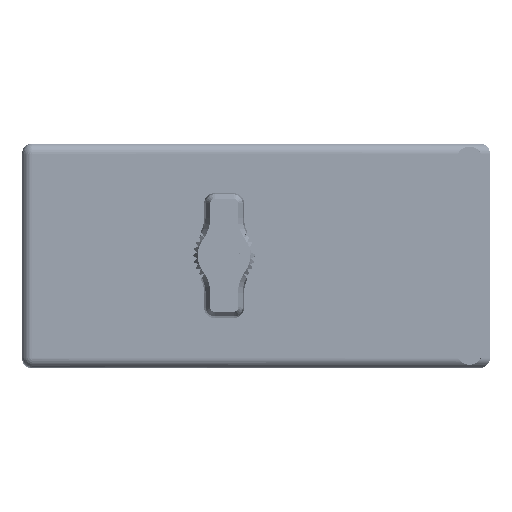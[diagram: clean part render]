
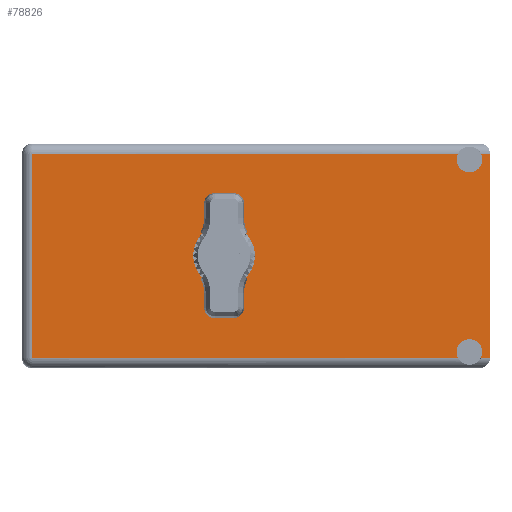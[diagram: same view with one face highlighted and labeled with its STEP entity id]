
A CAD part, top view. The second image highlights one B-rep face of the part: STEP entity #78826.
In plain terms, the highlighted face is planar.
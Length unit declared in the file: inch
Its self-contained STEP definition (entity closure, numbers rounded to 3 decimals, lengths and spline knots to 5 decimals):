
#187 = AXIS2_PLACEMENT_3D ( 'NONE', #57638, #48033, #14824 ) ;
#410 = CARTESIAN_POINT ( 'NONE',  ( 3.05, 2.03, -0.109 ) ) ;
#473 = VECTOR ( 'NONE', #90902, 39.37008 ) ;
#3218 = CARTESIAN_POINT ( 'NONE',  ( 2.97167, 2.03, -0.07 ) ) ;
#3903 = CARTESIAN_POINT ( 'NONE',  ( 3.19, 2.03, -0.07 ) ) ;
#4873 = CARTESIAN_POINT ( 'NONE',  ( 3.05, 2.03, -0.109 ) ) ;
#5989 = AXIS2_PLACEMENT_3D ( 'NONE', #103078, #86810, #69148 ) ;
#7048 = LINE ( 'NONE', #72676, #58517 ) ;
#9829 = DIRECTION ( 'NONE',  ( 1., 0., 0. ) ) ;
#10785 = DIRECTION ( 'NONE',  ( 0., 0., 1. ) ) ;
#13335 = DIRECTION ( 'NONE',  ( 0., 0., 1. ) ) ;
#13415 = VERTEX_POINT ( 'NONE', #73515 ) ;
#14133 = CIRCLE ( 'NONE', #187, 0.17 ) ;
#14623 = CIRCLE ( 'NONE', #77875, 0.0875 ) ;
#14824 = DIRECTION ( 'NONE',  ( 0., 0., 1. ) ) ;
#17156 = ORIENTED_EDGE ( 'NONE', *, *, #49502, .T. ) ;
#18059 = LINE ( 'NONE', #3903, #64268 ) ;
#18221 = VERTEX_POINT ( 'NONE', #25398 ) ;
#20281 = EDGE_CURVE ( 'NONE', #93238, #92271, #7048, .T. ) ;
#22033 = DIRECTION ( 'NONE',  ( 0., 0., 1. ) ) ;
#24570 = DIRECTION ( 'NONE',  ( 0., 1., 0. ) ) ;
#25398 = CARTESIAN_POINT ( 'NONE',  ( 1.3775, 2.03, -0.935 ) ) ;
#25740 = CARTESIAN_POINT ( 'NONE',  ( 2.97167, 2.03, -1.46 ) ) ;
#26006 = EDGE_CURVE ( 'NONE', #99739, #13415, #52169, .T. ) ;
#29541 = VERTEX_POINT ( 'NONE', #3218 ) ;
#31482 = CARTESIAN_POINT ( 'NONE',  ( 1.3775, 2.03, -0.595 ) ) ;
#32822 = CARTESIAN_POINT ( 'NONE',  ( 3.19, 2.03, -0.07 ) ) ;
#33106 = DIRECTION ( 'NONE',  ( 0., 1., 0. ) ) ;
#33468 = EDGE_CURVE ( 'NONE', #92677, #103857, #14623, .T. ) ;
#34198 = CARTESIAN_POINT ( 'NONE',  ( 3.19, 2.03, -0.07 ) ) ;
#34290 = ORIENTED_EDGE ( 'NONE', *, *, #36029, .F. ) ;
#36029 = EDGE_CURVE ( 'NONE', #13415, #29541, #36387, .T. ) ;
#36302 = AXIS2_PLACEMENT_3D ( 'NONE', #75220, #33106, #92182 ) ;
#36387 = CIRCLE ( 'NONE', #49057, 0.0875 ) ;
#36665 = EDGE_CURVE ( 'NONE', #18221, #41378, #106216, .T. ) ;
#36980 = DIRECTION ( 'NONE',  ( -1., 0., 0. ) ) ;
#37032 = CARTESIAN_POINT ( 'NONE',  ( 3.05, 2.03, -1.3335 ) ) ;
#37826 = DIRECTION ( 'NONE',  ( 1., 0., 0. ) ) ;
#40071 = CARTESIAN_POINT ( 'NONE',  ( 0.07, 2.03, -0.07 ) ) ;
#41191 = EDGE_LOOP ( 'NONE', ( #17156, #34290, #84764, #99276, #94895, #71056, #51616, #69160, #60393, #68053 ) ) ;
#41378 = VERTEX_POINT ( 'NONE', #31482 ) ;
#41881 = VECTOR ( 'NONE', #10785, 39.37008 ) ;
#44046 = AXIS2_PLACEMENT_3D ( 'NONE', #98160, #57509, #74173 ) ;
#45121 = CARTESIAN_POINT ( 'NONE',  ( 0., 2.03, -1.46 ) ) ;
#48033 = DIRECTION ( 'NONE',  ( 0., 1., 0. ) ) ;
#48607 = EDGE_CURVE ( 'NONE', #90953, #93238, #75284, .T. ) ;
#49057 = AXIS2_PLACEMENT_3D ( 'NONE', #410, #93023, #51255 ) ;
#49502 = EDGE_CURVE ( 'NONE', #92271, #29541, #81591, .T. ) ;
#49671 = CARTESIAN_POINT ( 'NONE',  ( 3.05, 2.03, -1.421 ) ) ;
#50411 = EDGE_CURVE ( 'NONE', #41378, #18221, #14133, .T. ) ;
#50850 = EDGE_CURVE ( 'NONE', #95085, #96416, #64353, .T. ) ;
#51255 = DIRECTION ( 'NONE',  ( 0., 0., 1. ) ) ;
#51616 = ORIENTED_EDGE ( 'NONE', *, *, #33468, .F. ) ;
#51783 = FACE_OUTER_BOUND ( 'NONE', #41191, .T. ) ;
#52169 = CIRCLE ( 'NONE', #99230, 0.0875 ) ;
#56058 = CARTESIAN_POINT ( 'NONE',  ( 0.07, 2.03, -1.46 ) ) ;
#57509 = DIRECTION ( 'NONE',  ( 0., 1., 0. ) ) ;
#57638 = CARTESIAN_POINT ( 'NONE',  ( 1.3775, 2.03, -0.765 ) ) ;
#58517 = VECTOR ( 'NONE', #22033, 39.37008 ) ;
#58681 = EDGE_LOOP ( 'NONE', ( #77665, #72167 ) ) ;
#60339 = CARTESIAN_POINT ( 'NONE',  ( 3.12833, 2.03, -0.07 ) ) ;
#60393 = ORIENTED_EDGE ( 'NONE', *, *, #48607, .T. ) ;
#63176 = VECTOR ( 'NONE', #9829, 39.37008 ) ;
#63917 = DIRECTION ( 'NONE',  ( 0., 1., 0. ) ) ;
#64268 = VECTOR ( 'NONE', #37826, 39.37008 ) ;
#64353 = LINE ( 'NONE', #103118, #41881 ) ;
#68053 = ORIENTED_EDGE ( 'NONE', *, *, #20281, .T. ) ;
#69148 = DIRECTION ( 'NONE',  ( 0., 0., 1. ) ) ;
#69160 = ORIENTED_EDGE ( 'NONE', *, *, #107006, .F. ) ;
#71056 = ORIENTED_EDGE ( 'NONE', *, *, #78273, .T. ) ;
#71354 = EDGE_CURVE ( 'NONE', #99739, #96416, #18059, .T. ) ;
#72167 = ORIENTED_EDGE ( 'NONE', *, *, #36665, .F. ) ;
#72676 = CARTESIAN_POINT ( 'NONE',  ( 0.07, 2.03, -1.53 ) ) ;
#73515 = CARTESIAN_POINT ( 'NONE',  ( 3.05, 2.03, -0.1965 ) ) ;
#73583 = CARTESIAN_POINT ( 'NONE',  ( 3.12833, 2.03, -1.46 ) ) ;
#74173 = DIRECTION ( 'NONE',  ( 0., 0., 1. ) ) ;
#75220 = CARTESIAN_POINT ( 'NONE',  ( 1.3775, 2.03, -0.765 ) ) ;
#75284 = LINE ( 'NONE', #45121, #99112 ) ;
#75439 = CARTESIAN_POINT ( 'NONE',  ( 3.19, 2.03, -1.46 ) ) ;
#77665 = ORIENTED_EDGE ( 'NONE', *, *, #50411, .F. ) ;
#77875 = AXIS2_PLACEMENT_3D ( 'NONE', #49671, #24570, #83646 ) ;
#78273 = EDGE_CURVE ( 'NONE', #95085, #103857, #102142, .T. ) ;
#78826 = ADVANCED_FACE ( 'NONE', ( #105946, #51783 ), #106634, .T. ) ;
#81591 = LINE ( 'NONE', #34198, #63176 ) ;
#83646 = DIRECTION ( 'NONE',  ( 0., 0., 1. ) ) ;
#83969 = CIRCLE ( 'NONE', #5989, 0.0875 ) ;
#84764 = ORIENTED_EDGE ( 'NONE', *, *, #26006, .F. ) ;
#86810 = DIRECTION ( 'NONE',  ( 0., 1., 0. ) ) ;
#90902 = DIRECTION ( 'NONE',  ( -1., 0., 0. ) ) ;
#90953 = VERTEX_POINT ( 'NONE', #25740 ) ;
#92182 = DIRECTION ( 'NONE',  ( 0., 0., 1. ) ) ;
#92271 = VERTEX_POINT ( 'NONE', #40071 ) ;
#92677 = VERTEX_POINT ( 'NONE', #37032 ) ;
#93023 = DIRECTION ( 'NONE',  ( 0., 1., 0. ) ) ;
#93238 = VERTEX_POINT ( 'NONE', #56058 ) ;
#94895 = ORIENTED_EDGE ( 'NONE', *, *, #50850, .F. ) ;
#95085 = VERTEX_POINT ( 'NONE', #75439 ) ;
#96416 = VERTEX_POINT ( 'NONE', #32822 ) ;
#98160 = CARTESIAN_POINT ( 'NONE',  ( 0., 2.03, -1.53 ) ) ;
#99112 = VECTOR ( 'NONE', #36980, 39.37008 ) ;
#99230 = AXIS2_PLACEMENT_3D ( 'NONE', #4873, #63917, #13335 ) ;
#99276 = ORIENTED_EDGE ( 'NONE', *, *, #71354, .T. ) ;
#99739 = VERTEX_POINT ( 'NONE', #60339 ) ;
#102142 = LINE ( 'NONE', #106772, #473 ) ;
#103078 = CARTESIAN_POINT ( 'NONE',  ( 3.05, 2.03, -1.421 ) ) ;
#103118 = CARTESIAN_POINT ( 'NONE',  ( 3.19, 2.03, 0. ) ) ;
#103857 = VERTEX_POINT ( 'NONE', #73583 ) ;
#105946 = FACE_BOUND ( 'NONE', #58681, .T. ) ;
#106216 = CIRCLE ( 'NONE', #36302, 0.17 ) ;
#106634 = PLANE ( 'NONE',  #44046 ) ;
#106772 = CARTESIAN_POINT ( 'NONE',  ( 0., 2.03, -1.46 ) ) ;
#107006 = EDGE_CURVE ( 'NONE', #90953, #92677, #83969, .T. ) ;
